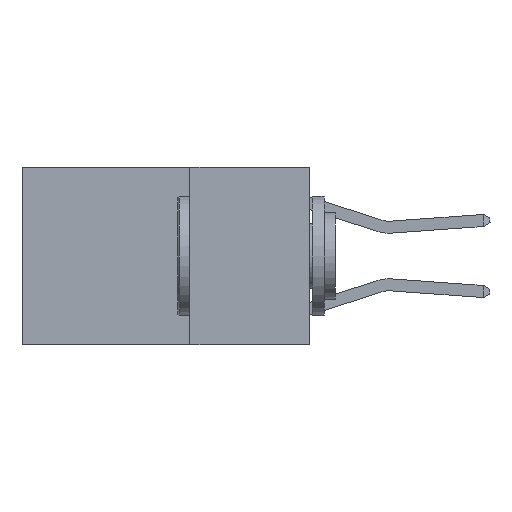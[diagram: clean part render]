
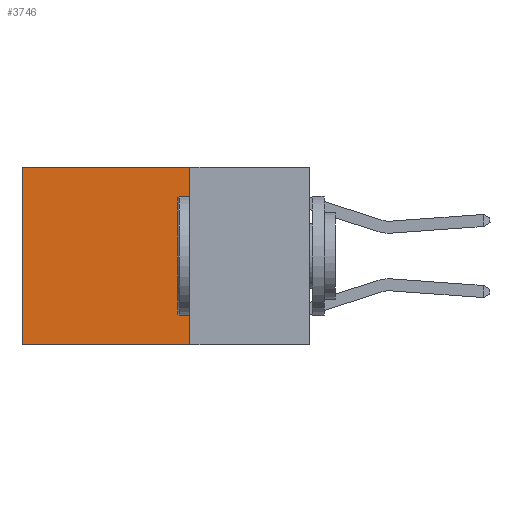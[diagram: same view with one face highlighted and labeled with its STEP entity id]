
A CAD part, left-side view. The second image highlights one B-rep face of the part: STEP entity #3746.
In plain terms, the highlighted planar face has unit normal (-1, 0, 0).
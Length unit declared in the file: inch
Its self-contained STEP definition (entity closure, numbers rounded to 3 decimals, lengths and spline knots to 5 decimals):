
#78 = EDGE_CURVE ( 'NONE', #973, #14813, #7085, .T. ) ;
#337 = VERTEX_POINT ( 'NONE', #14678 ) ;
#596 = FACE_OUTER_BOUND ( 'NONE', #13407, .T. ) ;
#677 = DIRECTION ( 'NONE',  ( 1., 0., 0. ) ) ;
#694 = EDGE_CURVE ( 'NONE', #8035, #337, #13555, .T. ) ;
#697 = LINE ( 'NONE', #10627, #13026 ) ;
#903 = DIRECTION ( 'NONE',  ( 0., 0., -1. ) ) ;
#973 = VERTEX_POINT ( 'NONE', #9158 ) ;
#1716 = CARTESIAN_POINT ( 'NONE',  ( 0.2625, 0.25, -0.37 ) ) ;
#1795 = DIRECTION ( 'NONE',  ( 0., 0., -1. ) ) ;
#2234 = ORIENTED_EDGE ( 'NONE', *, *, #694, .T. ) ;
#3589 = PLANE ( 'NONE',  #9954 ) ;
#3746 = ADVANCED_FACE ( 'NONE', ( #596 ), #3589, .F. ) ;
#3995 = CARTESIAN_POINT ( 'NONE',  ( 0.2625, 0.6, 0. ) ) ;
#4336 = CARTESIAN_POINT ( 'NONE',  ( 0.2625, 0.25, 0. ) ) ;
#4890 = DIRECTION ( 'NONE',  ( 0., 0., -1. ) ) ;
#6596 = VECTOR ( 'NONE', #4890, 39.37008 ) ;
#6662 = VECTOR ( 'NONE', #903, 39.37008 ) ;
#7085 = LINE ( 'NONE', #8150, #6662 ) ;
#8035 = VERTEX_POINT ( 'NONE', #3995 ) ;
#8150 = CARTESIAN_POINT ( 'NONE',  ( 0.2625, 0.25, 0. ) ) ;
#8164 = ORIENTED_EDGE ( 'NONE', *, *, #78, .F. ) ;
#8166 = DIRECTION ( 'NONE',  ( 0., 1., 0. ) ) ;
#9158 = CARTESIAN_POINT ( 'NONE',  ( 0.2625, 0.25, 0. ) ) ;
#9954 = AXIS2_PLACEMENT_3D ( 'NONE', #4336, #677, #1795 ) ;
#10627 = CARTESIAN_POINT ( 'NONE',  ( 0.2625, 0.25, 0. ) ) ;
#11093 = CARTESIAN_POINT ( 'NONE',  ( 0.2625, 0.6, 0. ) ) ;
#12059 = ORIENTED_EDGE ( 'NONE', *, *, #12900, .T. ) ;
#12900 = EDGE_CURVE ( 'NONE', #973, #8035, #697, .T. ) ;
#13026 = VECTOR ( 'NONE', #15566, 39.37008 ) ;
#13261 = CARTESIAN_POINT ( 'NONE',  ( 0.2625, 0.25, -0.37 ) ) ;
#13407 = EDGE_LOOP ( 'NONE', ( #2234, #13719, #8164, #12059 ) ) ;
#13555 = LINE ( 'NONE', #11093, #6596 ) ;
#13719 = ORIENTED_EDGE ( 'NONE', *, *, #14416, .F. ) ;
#14109 = VECTOR ( 'NONE', #8166, 39.37008 ) ;
#14416 = EDGE_CURVE ( 'NONE', #14813, #337, #15786, .T. ) ;
#14678 = CARTESIAN_POINT ( 'NONE',  ( 0.2625, 0.6, -0.37 ) ) ;
#14813 = VERTEX_POINT ( 'NONE', #13261 ) ;
#15566 = DIRECTION ( 'NONE',  ( 0., 1., 0. ) ) ;
#15786 = LINE ( 'NONE', #1716, #14109 ) ;
